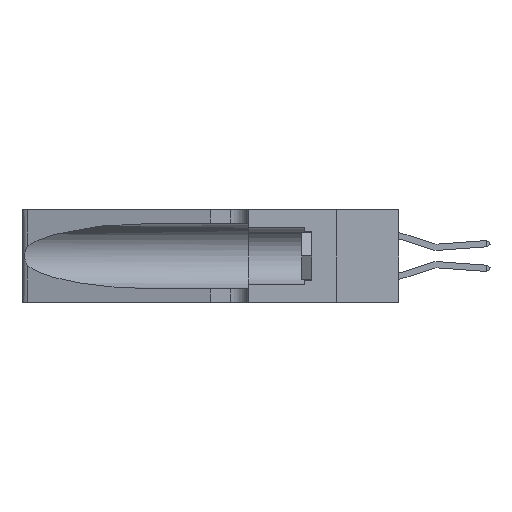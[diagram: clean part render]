
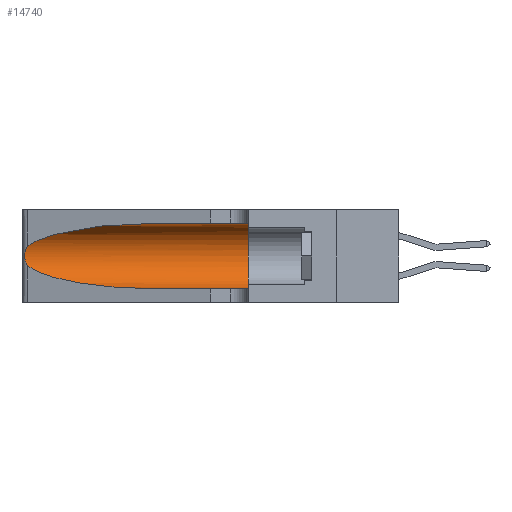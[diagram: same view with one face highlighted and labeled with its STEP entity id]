
A CAD part, left-side view. The second image highlights one B-rep face of the part: STEP entity #14740.
In plain terms, the highlighted cylindrical face has radius 3.308 mm (diameter 6.617 mm), a partial arc.
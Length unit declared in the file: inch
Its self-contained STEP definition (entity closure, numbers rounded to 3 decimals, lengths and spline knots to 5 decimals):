
#573 = CARTESIAN_POINT ( 'NONE',  ( 0.25639, 1.23186, 0.15144 ) ) ;
#715 = CARTESIAN_POINT ( 'NONE',  ( 0.26075, 1.23896, 0.178 ) ) ;
#2122 = CARTESIAN_POINT ( 'NONE',  ( 0.2373, 1.15595, 0.28018 ) ) ;
#2664 = VERTEX_POINT ( 'NONE', #28642 ) ;
#3888 = CARTESIAN_POINT ( 'NONE',  ( 0.26075, 1.23896, 0.19203 ) ) ;
#4026 = CARTESIAN_POINT ( 'NONE',  ( 0.25555, 1.22993, 0.14849 ) ) ;
#4130 = VERTEX_POINT ( 'NONE', #9965 ) ;
#5162 = CARTESIAN_POINT ( 'NONE',  ( 0.25487, 1.22718, 0.22369 ) ) ;
#6276 = CARTESIAN_POINT ( 'NONE',  ( 0.25854, 1.2359, 0.20912 ) ) ;
#6778 = CARTESIAN_POINT ( 'NONE',  ( 0.2373, 1.15595, 0.08982 ) ) ;
#6969 = VERTEX_POINT ( 'NONE', #17550 ) ;
#7274 = VECTOR ( 'NONE', #21213, 39.37008 ) ;
#7343 = FACE_OUTER_BOUND ( 'NONE', #17011, .T. ) ;
#7447 =( BOUNDED_CURVE ( )  B_SPLINE_CURVE ( 3, ( #11439, #21304, #2122, #5162 ),
 .UNSPECIFIED., .F., .F. ) 
 B_SPLINE_CURVE_WITH_KNOTS ( ( 4, 4 ),
 ( 1.5708, 2.84003 ),
 .UNSPECIFIED. ) 
 CURVE ( )  GEOMETRIC_REPRESENTATION_ITEM ( )  RATIONAL_B_SPLINE_CURVE ( ( 1., 0.87, 0.87, 1. ) ) 
 REPRESENTATION_ITEM ( '' )  );
#8362 = LINE ( 'NONE', #8810, #15816 ) ;
#8810 = CARTESIAN_POINT ( 'NONE',  ( 0.1305, 1.61858, 0.05475 ) ) ;
#9965 = CARTESIAN_POINT ( 'NONE',  ( 0.1305, 0.72297, 0.05475 ) ) ;
#10151 = CARTESIAN_POINT ( 'NONE',  ( 0.26017, 1.23833, 0.17102 ) ) ;
#10373 = DIRECTION ( 'NONE',  ( 0., 0., 1. ) ) ;
#10380 = ORIENTED_EDGE ( 'NONE', *, *, #20748, .T. ) ;
#10450 = CARTESIAN_POINT ( 'NONE',  ( 0.26018, 1.23835, 0.19895 ) ) ;
#11046 = EDGE_CURVE ( 'NONE', #2664, #22492, #24218, .T. ) ;
#11216 = ORIENTED_EDGE ( 'NONE', *, *, #11046, .F. ) ;
#11439 = CARTESIAN_POINT ( 'NONE',  ( 0.1305, 0.72297, 0.31525 ) ) ;
#11986 = DIRECTION ( 'NONE',  ( 0., -1., 0. ) ) ;
#14740 = ADVANCED_FACE ( 'NONE', ( #7343 ), #23762, .F. ) ;
#15816 = VECTOR ( 'NONE', #37343, 39.37008 ) ;
#16004 = CARTESIAN_POINT ( 'NONE',  ( 0.18966, 0.96281, 0.05475 ) ) ;
#16692 = CARTESIAN_POINT ( 'NONE',  ( 0.25487, 1.22718, 0.14631 ) ) ;
#16813 = ORIENTED_EDGE ( 'NONE', *, *, #27723, .T. ) ;
#17011 = EDGE_LOOP ( 'NONE', ( #31216, #18562, #10380, #16813, #36915, #11216 ) ) ;
#17550 = CARTESIAN_POINT ( 'NONE',  ( 0.25487, 1.22718, 0.14631 ) ) ;
#18326 = AXIS2_PLACEMENT_3D ( 'NONE', #24782, #11986, #34163 ) ;
#18562 = ORIENTED_EDGE ( 'NONE', *, *, #23384, .T. ) ;
#20748 = EDGE_CURVE ( 'NONE', #6969, #4130, #22208, .T. ) ;
#21213 = DIRECTION ( 'NONE',  ( 0., -1., 0. ) ) ;
#21304 = CARTESIAN_POINT ( 'NONE',  ( 0.18966, 0.96281, 0.31525 ) ) ;
#21588 = CARTESIAN_POINT ( 'NONE',  ( 0.25487, 1.22718, 0.14631 ) ) ;
#22208 =( BOUNDED_CURVE ( )  B_SPLINE_CURVE ( 3, ( #21588, #6778, #16004, #22366 ),
 .UNSPECIFIED., .F., .F. ) 
 B_SPLINE_CURVE_WITH_KNOTS ( ( 4, 4 ),
 ( 3.44316, 4.71239 ),
 .UNSPECIFIED. ) 
 CURVE ( )  GEOMETRIC_REPRESENTATION_ITEM ( )  RATIONAL_B_SPLINE_CURVE ( ( 1., 0.87, 0.87, 1. ) ) 
 REPRESENTATION_ITEM ( '' )  );
#22366 = CARTESIAN_POINT ( 'NONE',  ( 0.1305, 0.72297, 0.05475 ) ) ;
#22492 = VERTEX_POINT ( 'NONE', #30132 ) ;
#22597 = CARTESIAN_POINT ( 'NONE',  ( 0.1305, 0.35, 0.185 ) ) ;
#23375 = CARTESIAN_POINT ( 'NONE',  ( 0.25789, 1.23486, 0.15765 ) ) ;
#23384 = EDGE_CURVE ( 'NONE', #26714, #6969, #34386, .T. ) ;
#23762 = CYLINDRICAL_SURFACE ( 'NONE', #18326, 0.13025 ) ;
#23853 = CARTESIAN_POINT ( 'NONE',  ( 0.1305, 1.61858, 0.31525 ) ) ;
#24218 = LINE ( 'NONE', #23853, #7274 ) ;
#24782 = CARTESIAN_POINT ( 'NONE',  ( 0.1305, 1.61858, 0.185 ) ) ;
#26255 = CARTESIAN_POINT ( 'NONE',  ( 0.1305, 0.35, 0.05475 ) ) ;
#26406 = EDGE_CURVE ( 'NONE', #2664, #26714, #7447, .T. ) ;
#26714 = VERTEX_POINT ( 'NONE', #31984 ) ;
#27095 = EDGE_CURVE ( 'NONE', #22492, #27599, #31055, .T. ) ;
#27599 = VERTEX_POINT ( 'NONE', #26255 ) ;
#27723 = EDGE_CURVE ( 'NONE', #4130, #27599, #8362, .T. ) ;
#28642 = CARTESIAN_POINT ( 'NONE',  ( 0.1305, 0.72297, 0.31525 ) ) ;
#28990 = CARTESIAN_POINT ( 'NONE',  ( 0.25555, 1.22994, 0.2215 ) ) ;
#30132 = CARTESIAN_POINT ( 'NONE',  ( 0.1305, 0.35, 0.31525 ) ) ;
#31055 = CIRCLE ( 'NONE', #38574, 0.13025 ) ;
#31216 = ORIENTED_EDGE ( 'NONE', *, *, #26406, .T. ) ;
#31984 = CARTESIAN_POINT ( 'NONE',  ( 0.25487, 1.22718, 0.22369 ) ) ;
#32929 = CARTESIAN_POINT ( 'NONE',  ( 0.25856, 1.23593, 0.16098 ) ) ;
#34163 = DIRECTION ( 'NONE',  ( 0., 0., -1. ) ) ;
#34386 = B_SPLINE_CURVE_WITH_KNOTS ( 'NONE', 3,
 ( #35261, #28990, #34849, #38570, #6276, #10450, #3888, #715, #10151, #32929, #23375, #573, #4026, #16692 ),
 .UNSPECIFIED., .F., .F.,
 ( 4, 2, 2, 2, 2, 2, 4 ),
 ( 0., 0.00027, 0.00053, 0.00107, 0.0016, 0.00187, 0.00214 ),
 .UNSPECIFIED. ) ;
#34849 = CARTESIAN_POINT ( 'NONE',  ( 0.25639, 1.23184, 0.21858 ) ) ;
#35196 = DIRECTION ( 'NONE',  ( 0., 1., 0. ) ) ;
#35261 = CARTESIAN_POINT ( 'NONE',  ( 0.25487, 1.22718, 0.22369 ) ) ;
#36915 = ORIENTED_EDGE ( 'NONE', *, *, #27095, .F. ) ;
#37343 = DIRECTION ( 'NONE',  ( 0., -1., 0. ) ) ;
#38570 = CARTESIAN_POINT ( 'NONE',  ( 0.25787, 1.23484, 0.2124 ) ) ;
#38574 = AXIS2_PLACEMENT_3D ( 'NONE', #22597, #35196, #10373 ) ;
